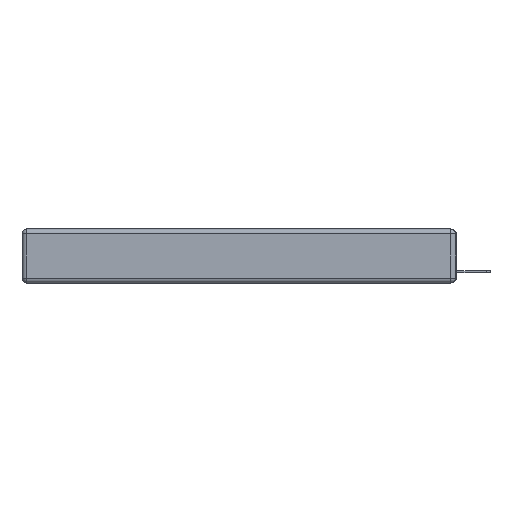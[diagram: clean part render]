
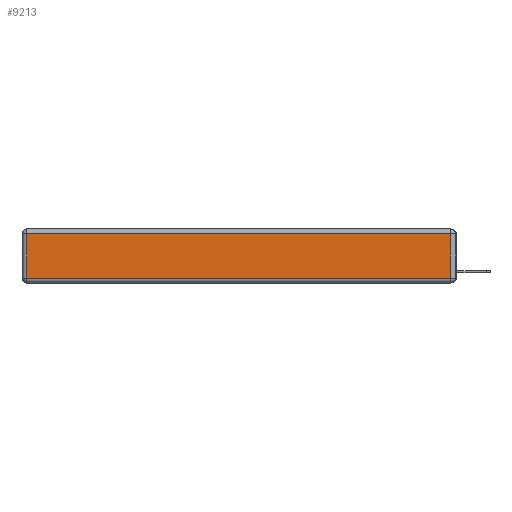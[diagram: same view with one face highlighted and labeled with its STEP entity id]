
A CAD part, left-side view. The second image highlights one B-rep face of the part: STEP entity #9213.
In plain terms, the highlighted planar face has unit normal (-1, 0, 0).
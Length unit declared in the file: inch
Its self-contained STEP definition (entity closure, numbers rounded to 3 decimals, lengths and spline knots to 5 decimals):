
#1746 = VERTEX_POINT ( 'NONE', #22303 ) ;
#3825 = ORIENTED_EDGE ( 'NONE', *, *, #23892, .T. ) ;
#4058 = VECTOR ( 'NONE', #4914, 39.37008 ) ;
#4914 = DIRECTION ( 'NONE',  ( 0., 1., 0. ) ) ;
#4999 = CARTESIAN_POINT ( 'NONE',  ( 0., 2.75, -0.03 ) ) ;
#5122 = DIRECTION ( 'NONE',  ( -1., 0., 0. ) ) ;
#5166 = EDGE_CURVE ( 'NONE', #6012, #6072, #14226, .T. ) ;
#5726 = CARTESIAN_POINT ( 'NONE',  ( 0., 2.72, -0.343 ) ) ;
#6012 = VERTEX_POINT ( 'NONE', #20469 ) ;
#6072 = VERTEX_POINT ( 'NONE', #17898 ) ;
#7114 = VECTOR ( 'NONE', #8132, 39.37008 ) ;
#7781 = ORIENTED_EDGE ( 'NONE', *, *, #5166, .T. ) ;
#8132 = DIRECTION ( 'NONE',  ( 0., 0., 1. ) ) ;
#8459 = VERTEX_POINT ( 'NONE', #9537 ) ;
#8823 = AXIS2_PLACEMENT_3D ( 'NONE', #11084, #5122, #23329 ) ;
#8953 = DIRECTION ( 'NONE',  ( 0., -1., 0. ) ) ;
#9120 = PLANE ( 'NONE',  #8823 ) ;
#9213 = ADVANCED_FACE ( 'NONE', ( #25119 ), #9120, .T. ) ;
#9537 = CARTESIAN_POINT ( 'NONE',  ( 0., 0.03, -0.313 ) ) ;
#10314 = VECTOR ( 'NONE', #19904, 39.37008 ) ;
#11005 = CARTESIAN_POINT ( 'NONE',  ( 0., 0., -0.313 ) ) ;
#11084 = CARTESIAN_POINT ( 'NONE',  ( 0., 0., -0.343 ) ) ;
#11290 = ORIENTED_EDGE ( 'NONE', *, *, #24400, .T. ) ;
#12058 = CARTESIAN_POINT ( 'NONE',  ( 0., 0.03, -0.343 ) ) ;
#12817 = VECTOR ( 'NONE', #8953, 39.37008 ) ;
#13139 = LINE ( 'NONE', #11005, #12817 ) ;
#14028 = EDGE_LOOP ( 'NONE', ( #24989, #3825, #7781, #11290 ) ) ;
#14226 = LINE ( 'NONE', #4999, #4058 ) ;
#14461 = LINE ( 'NONE', #12058, #7114 ) ;
#17898 = CARTESIAN_POINT ( 'NONE',  ( 0., 2.72, -0.03 ) ) ;
#17950 = EDGE_CURVE ( 'NONE', #1746, #8459, #13139, .T. ) ;
#19509 = LINE ( 'NONE', #5726, #10314 ) ;
#19904 = DIRECTION ( 'NONE',  ( 0., 0., -1. ) ) ;
#20469 = CARTESIAN_POINT ( 'NONE',  ( 0., 0.03, -0.03 ) ) ;
#22303 = CARTESIAN_POINT ( 'NONE',  ( 0., 2.72, -0.313 ) ) ;
#23329 = DIRECTION ( 'NONE',  ( 0., 0., 1. ) ) ;
#23892 = EDGE_CURVE ( 'NONE', #8459, #6012, #14461, .T. ) ;
#24400 = EDGE_CURVE ( 'NONE', #6072, #1746, #19509, .T. ) ;
#24989 = ORIENTED_EDGE ( 'NONE', *, *, #17950, .T. ) ;
#25119 = FACE_OUTER_BOUND ( 'NONE', #14028, .T. ) ;
